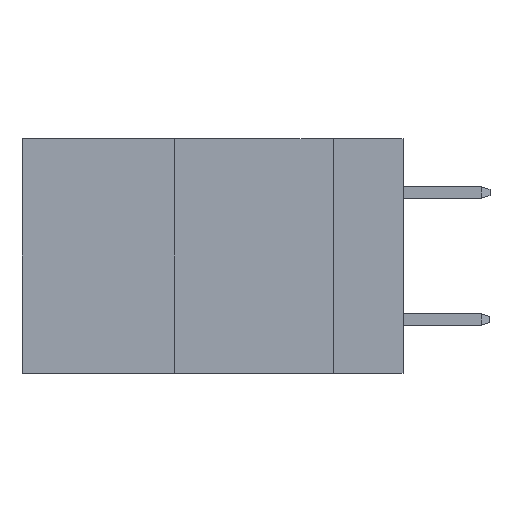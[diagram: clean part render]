
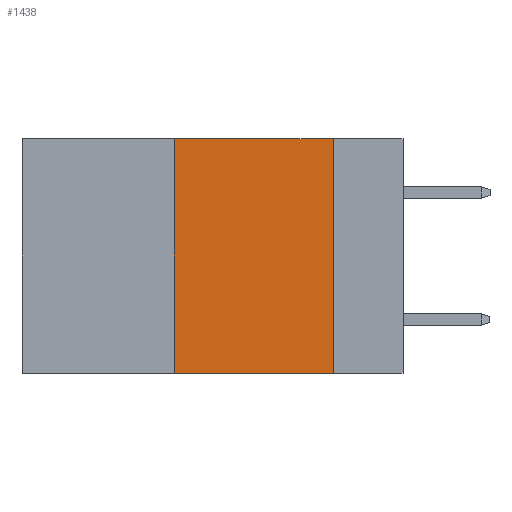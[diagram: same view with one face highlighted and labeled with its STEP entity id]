
A CAD part, left-side view. The second image highlights one B-rep face of the part: STEP entity #1438.
In plain terms, the highlighted planar face has unit normal (-1, 0, 0).
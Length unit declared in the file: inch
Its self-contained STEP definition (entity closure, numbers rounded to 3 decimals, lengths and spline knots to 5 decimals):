
#125 = ORIENTED_EDGE ( 'NONE', *, *, #8495, .F. ) ;
#1162 = EDGE_CURVE ( 'NONE', #1352, #7235, #2180, .T. ) ;
#1173 = CARTESIAN_POINT ( 'NONE',  ( 0., 0.6, -0.37 ) ) ;
#1328 = FACE_OUTER_BOUND ( 'NONE', #5822, .T. ) ;
#1352 = VERTEX_POINT ( 'NONE', #7720 ) ;
#1438 = ADVANCED_FACE ( 'NONE', ( #1328 ), #11165, .F. ) ;
#2029 = DIRECTION ( 'NONE',  ( 1., 0., 0. ) ) ;
#2039 = CARTESIAN_POINT ( 'NONE',  ( 0., 0.11, 0. ) ) ;
#2180 = LINE ( 'NONE', #8453, #4494 ) ;
#2271 = VERTEX_POINT ( 'NONE', #4823 ) ;
#2786 = AXIS2_PLACEMENT_3D ( 'NONE', #3836, #2029, #10336 ) ;
#3415 = VECTOR ( 'NONE', #5489, 39.37008 ) ;
#3836 = CARTESIAN_POINT ( 'NONE',  ( 0., 0.6, 0. ) ) ;
#3848 = DIRECTION ( 'NONE',  ( 0., -1., 0. ) ) ;
#4494 = VECTOR ( 'NONE', #11134, 39.37008 ) ;
#4745 = EDGE_CURVE ( 'NONE', #1352, #9732, #9151, .T. ) ;
#4795 = ORIENTED_EDGE ( 'NONE', *, *, #4745, .T. ) ;
#4822 = EDGE_CURVE ( 'NONE', #2271, #9732, #8373, .T. ) ;
#4823 = CARTESIAN_POINT ( 'NONE',  ( 0., 0.11, 0. ) ) ;
#5489 = DIRECTION ( 'NONE',  ( 0., -1., 0. ) ) ;
#5822 = EDGE_LOOP ( 'NONE', ( #6878, #125, #9309, #4795 ) ) ;
#6878 = ORIENTED_EDGE ( 'NONE', *, *, #4822, .F. ) ;
#7235 = VERTEX_POINT ( 'NONE', #9253 ) ;
#7275 = LINE ( 'NONE', #9978, #3415 ) ;
#7720 = CARTESIAN_POINT ( 'NONE',  ( 0., 0.36, -0.37 ) ) ;
#8373 = LINE ( 'NONE', #2039, #9856 ) ;
#8453 = CARTESIAN_POINT ( 'NONE',  ( 0., 0.36, 0. ) ) ;
#8495 = EDGE_CURVE ( 'NONE', #7235, #2271, #7275, .T. ) ;
#8678 = CARTESIAN_POINT ( 'NONE',  ( 0., 0.11, -0.37 ) ) ;
#9151 = LINE ( 'NONE', #1173, #10217 ) ;
#9253 = CARTESIAN_POINT ( 'NONE',  ( 0., 0.36, 0. ) ) ;
#9309 = ORIENTED_EDGE ( 'NONE', *, *, #1162, .F. ) ;
#9732 = VERTEX_POINT ( 'NONE', #8678 ) ;
#9856 = VECTOR ( 'NONE', #10184, 39.37008 ) ;
#9978 = CARTESIAN_POINT ( 'NONE',  ( 0., 0.6, 0. ) ) ;
#10184 = DIRECTION ( 'NONE',  ( 0., 0., -1. ) ) ;
#10217 = VECTOR ( 'NONE', #3848, 39.37008 ) ;
#10336 = DIRECTION ( 'NONE',  ( 0., 0., -1. ) ) ;
#11134 = DIRECTION ( 'NONE',  ( 0., 0., 1. ) ) ;
#11165 = PLANE ( 'NONE',  #2786 ) ;
